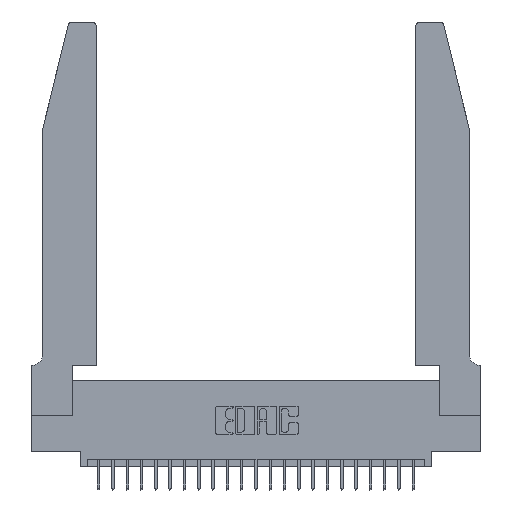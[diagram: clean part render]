
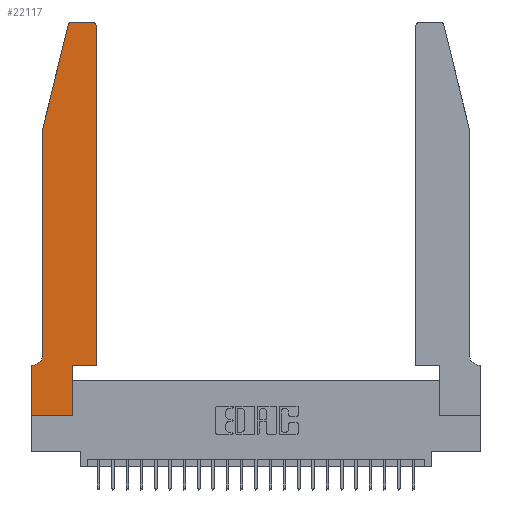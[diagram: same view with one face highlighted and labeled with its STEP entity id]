
A CAD part, top view. The second image highlights one B-rep face of the part: STEP entity #22117.
In plain terms, the highlighted planar face has unit normal (0, 0, 1).
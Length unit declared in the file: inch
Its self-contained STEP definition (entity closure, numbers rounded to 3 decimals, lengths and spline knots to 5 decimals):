
#412 = LINE ( 'NONE', #626, #5682 ) ;
#467 = EDGE_CURVE ( 'NONE', #17433, #22852, #905, .T. ) ;
#626 = CARTESIAN_POINT ( 'NONE',  ( 0.2865, 0.35, 0.37 ) ) ;
#905 = CIRCLE ( 'NONE', #9836, 0.03 ) ;
#1517 = EDGE_CURVE ( 'NONE', #14286, #3894, #19453, .T. ) ;
#1837 = AXIS2_PLACEMENT_3D ( 'NONE', #22360, #10600, #24325 ) ;
#1930 = VECTOR ( 'NONE', #9081, 39.37008 ) ;
#2150 = CARTESIAN_POINT ( 'NONE',  ( 0.2605, 2.75, 0.37 ) ) ;
#2299 = CARTESIAN_POINT ( 'NONE',  ( 0.0755, 0.42, 0.37 ) ) ;
#2517 = DIRECTION ( 'NONE',  ( 1., 0., 0. ) ) ;
#2758 = ORIENTED_EDGE ( 'NONE', *, *, #3014, .T. ) ;
#2764 = AXIS2_PLACEMENT_3D ( 'NONE', #6828, #20647, #8857 ) ;
#3014 = EDGE_CURVE ( 'NONE', #22852, #25147, #3142, .T. ) ;
#3142 = LINE ( 'NONE', #2150, #23520 ) ;
#3206 = LINE ( 'NONE', #20614, #12541 ) ;
#3237 = ORIENTED_EDGE ( 'NONE', *, *, #5157, .T. ) ;
#3294 = DIRECTION ( 'NONE',  ( 0., 1., 0. ) ) ;
#3475 = CARTESIAN_POINT ( 'NONE',  ( 0.4205, 2.75, 0.37 ) ) ;
#3612 = FACE_OUTER_BOUND ( 'NONE', #8774, .T. ) ;
#3894 = VERTEX_POINT ( 'NONE', #19093 ) ;
#3906 = DIRECTION ( 'NONE',  ( 0., -1., 0. ) ) ;
#5157 = EDGE_CURVE ( 'NONE', #12626, #11200, #9638, .T. ) ;
#5682 = VECTOR ( 'NONE', #22320, 39.37008 ) ;
#5853 = DIRECTION ( 'NONE',  ( -0.239, -0.971, 0. ) ) ;
#6505 = EDGE_CURVE ( 'NONE', #17723, #19408, #23083, .T. ) ;
#6828 = CARTESIAN_POINT ( 'NONE',  ( 0.0055, 0.42, 0.37 ) ) ;
#6962 = PLANE ( 'NONE',  #11954 ) ;
#7280 = CARTESIAN_POINT ( 'NONE',  ( 0.4505, 0.35, 0.37 ) ) ;
#7623 = CARTESIAN_POINT ( 'NONE',  ( 0.0755, 2., 0.37 ) ) ;
#7702 = CIRCLE ( 'NONE', #2764, 0.07 ) ;
#7763 = ORIENTED_EDGE ( 'NONE', *, *, #21214, .T. ) ;
#8668 = EDGE_CURVE ( 'NONE', #3894, #12626, #412, .T. ) ;
#8774 = EDGE_LOOP ( 'NONE', ( #2758, #20404, #7763, #13073, #21973, #17996, #14004, #14988, #14059, #3237, #16910, #17815 ) ) ;
#8810 = CARTESIAN_POINT ( 'NONE',  ( 0.4505, 2.72, 0.37 ) ) ;
#8832 = EDGE_CURVE ( 'NONE', #19854, #11144, #22361, .T. ) ;
#8857 = DIRECTION ( 'NONE',  ( -1., 0., 0. ) ) ;
#9081 = DIRECTION ( 'NONE',  ( -1., 0., 0. ) ) ;
#9638 = LINE ( 'NONE', #25528, #20105 ) ;
#9821 = EDGE_CURVE ( 'NONE', #19408, #19854, #7702, .T. ) ;
#9831 = DIRECTION ( 'NONE',  ( 1., 0., 0. ) ) ;
#9836 = AXIS2_PLACEMENT_3D ( 'NONE', #22006, #16882, #25049 ) ;
#10600 = DIRECTION ( 'NONE',  ( 0., 0., 1. ) ) ;
#10936 = CARTESIAN_POINT ( 'NONE',  ( 0.284, 2.75, 0.37 ) ) ;
#10988 = DIRECTION ( 'NONE',  ( 0., 0., 1. ) ) ;
#11116 = VECTOR ( 'NONE', #5853, 39.37008 ) ;
#11144 = VERTEX_POINT ( 'NONE', #16272 ) ;
#11200 = VERTEX_POINT ( 'NONE', #24549 ) ;
#11321 = CARTESIAN_POINT ( 'NONE',  ( 0., 0., 0.37 ) ) ;
#11954 = AXIS2_PLACEMENT_3D ( 'NONE', #18806, #10988, #24692 ) ;
#12541 = VECTOR ( 'NONE', #18643, 39.37008 ) ;
#12626 = VERTEX_POINT ( 'NONE', #21228 ) ;
#13073 = ORIENTED_EDGE ( 'NONE', *, *, #6505, .T. ) ;
#14004 = ORIENTED_EDGE ( 'NONE', *, *, #17428, .T. ) ;
#14059 = ORIENTED_EDGE ( 'NONE', *, *, #8668, .T. ) ;
#14286 = VERTEX_POINT ( 'NONE', #11321 ) ;
#14988 = ORIENTED_EDGE ( 'NONE', *, *, #1517, .T. ) ;
#15114 = EDGE_CURVE ( 'NONE', #25147, #20827, #20119, .T. ) ;
#15498 = CARTESIAN_POINT ( 'NONE',  ( 0.0055, 0.35, 0.37 ) ) ;
#16272 = CARTESIAN_POINT ( 'NONE',  ( 0., 0.35, 0.37 ) ) ;
#16882 = DIRECTION ( 'NONE',  ( 0., 0., 1. ) ) ;
#16910 = ORIENTED_EDGE ( 'NONE', *, *, #24628, .T. ) ;
#17428 = EDGE_CURVE ( 'NONE', #11144, #14286, #3206, .T. ) ;
#17433 = VERTEX_POINT ( 'NONE', #8810 ) ;
#17723 = VERTEX_POINT ( 'NONE', #7623 ) ;
#17815 = ORIENTED_EDGE ( 'NONE', *, *, #467, .T. ) ;
#17996 = ORIENTED_EDGE ( 'NONE', *, *, #8832, .T. ) ;
#18016 = DIRECTION ( 'NONE',  ( -1., 0., 0. ) ) ;
#18615 = CARTESIAN_POINT ( 'NONE',  ( 0.25487, 2.72718, 0.37 ) ) ;
#18643 = DIRECTION ( 'NONE',  ( 0., -1., 0. ) ) ;
#18806 = CARTESIAN_POINT ( 'NONE',  ( 0., 0.35, 0.37 ) ) ;
#19093 = CARTESIAN_POINT ( 'NONE',  ( 0.2865, 0., 0.37 ) ) ;
#19408 = VERTEX_POINT ( 'NONE', #2299 ) ;
#19453 = LINE ( 'NONE', #24438, #25245 ) ;
#19854 = VERTEX_POINT ( 'NONE', #15498 ) ;
#20105 = VECTOR ( 'NONE', #9831, 39.37008 ) ;
#20119 = CIRCLE ( 'NONE', #1837, 0.03 ) ;
#20404 = ORIENTED_EDGE ( 'NONE', *, *, #15114, .T. ) ;
#20614 = CARTESIAN_POINT ( 'NONE',  ( 0., 0., 0.37 ) ) ;
#20647 = DIRECTION ( 'NONE',  ( 0., 0., -1. ) ) ;
#20827 = VERTEX_POINT ( 'NONE', #18615 ) ;
#21181 = VECTOR ( 'NONE', #3294, 39.37008 ) ;
#21214 = EDGE_CURVE ( 'NONE', #20827, #17723, #22168, .T. ) ;
#21228 = CARTESIAN_POINT ( 'NONE',  ( 0.2865, 0.35, 0.37 ) ) ;
#21578 = CARTESIAN_POINT ( 'NONE',  ( 0.0755, 2., 0.37 ) ) ;
#21973 = ORIENTED_EDGE ( 'NONE', *, *, #9821, .T. ) ;
#22006 = CARTESIAN_POINT ( 'NONE',  ( 0.4205, 2.72, 0.37 ) ) ;
#22117 = ADVANCED_FACE ( 'NONE', ( #3612 ), #6962, .T. ) ;
#22168 = LINE ( 'NONE', #21578, #11116 ) ;
#22320 = DIRECTION ( 'NONE',  ( 0., 1., 0. ) ) ;
#22360 = CARTESIAN_POINT ( 'NONE',  ( 0.284, 2.72, 0.37 ) ) ;
#22361 = LINE ( 'NONE', #22835, #1930 ) ;
#22476 = VECTOR ( 'NONE', #3906, 39.37008 ) ;
#22835 = CARTESIAN_POINT ( 'NONE',  ( 0.0755, 0.35, 0.37 ) ) ;
#22852 = VERTEX_POINT ( 'NONE', #3475 ) ;
#23018 = LINE ( 'NONE', #7280, #21181 ) ;
#23083 = LINE ( 'NONE', #25553, #22476 ) ;
#23520 = VECTOR ( 'NONE', #18016, 39.37008 ) ;
#24325 = DIRECTION ( 'NONE',  ( 1., 0., 0. ) ) ;
#24438 = CARTESIAN_POINT ( 'NONE',  ( 0., 0., 0.37 ) ) ;
#24549 = CARTESIAN_POINT ( 'NONE',  ( 0.4505, 0.35, 0.37 ) ) ;
#24628 = EDGE_CURVE ( 'NONE', #11200, #17433, #23018, .T. ) ;
#24692 = DIRECTION ( 'NONE',  ( 1., 0., 0. ) ) ;
#25049 = DIRECTION ( 'NONE',  ( 1., 0., 0. ) ) ;
#25147 = VERTEX_POINT ( 'NONE', #10936 ) ;
#25245 = VECTOR ( 'NONE', #2517, 39.37008 ) ;
#25528 = CARTESIAN_POINT ( 'NONE',  ( 0.4505, 0.35, 0.37 ) ) ;
#25553 = CARTESIAN_POINT ( 'NONE',  ( 0.0755, 2., 0.37 ) ) ;
